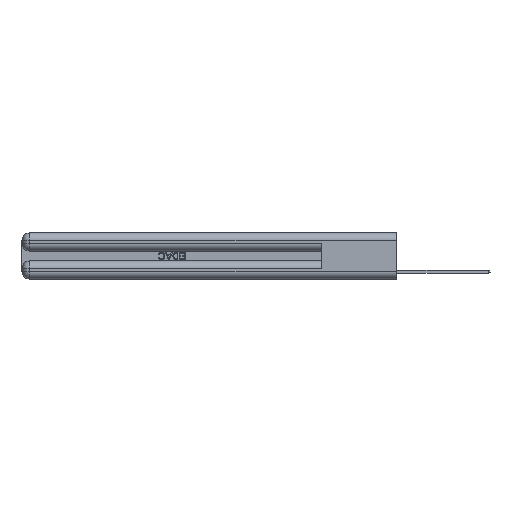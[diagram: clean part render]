
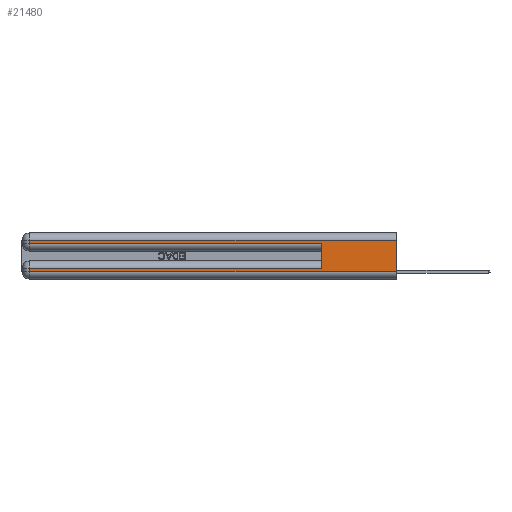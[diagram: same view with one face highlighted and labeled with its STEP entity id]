
A CAD part, left-side view. The second image highlights one B-rep face of the part: STEP entity #21480.
In plain terms, the highlighted planar face has unit normal (-1, 0, 0).
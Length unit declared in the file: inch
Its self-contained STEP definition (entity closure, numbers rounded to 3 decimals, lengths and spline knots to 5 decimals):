
#236 = CARTESIAN_POINT ( 'NONE',  ( 0., 2.94, 0.31 ) ) ;
#272 = EDGE_CURVE ( 'NONE', #16453, #19602, #9130, .T. ) ;
#356 = EDGE_CURVE ( 'NONE', #14904, #26834, #14768, .T. ) ;
#558 = CARTESIAN_POINT ( 'NONE',  ( 0., 0., 0.06 ) ) ;
#974 = VECTOR ( 'NONE', #5524, 39.37008 ) ;
#1012 = LINE ( 'NONE', #23505, #15067 ) ;
#1538 = EDGE_LOOP ( 'NONE', ( #4612, #5909, #6486, #6967, #2007, #4223, #28907, #12622 ) ) ;
#1742 = VECTOR ( 'NONE', #5453, 39.37008 ) ;
#2007 = ORIENTED_EDGE ( 'NONE', *, *, #27892, .F. ) ;
#2695 = VERTEX_POINT ( 'NONE', #4060 ) ;
#4060 = CARTESIAN_POINT ( 'NONE',  ( 0., 0., 0.31 ) ) ;
#4223 = ORIENTED_EDGE ( 'NONE', *, *, #356, .T. ) ;
#4612 = ORIENTED_EDGE ( 'NONE', *, *, #16664, .F. ) ;
#4970 = CARTESIAN_POINT ( 'NONE',  ( 0., 2.94, 0.37 ) ) ;
#5013 = CARTESIAN_POINT ( 'NONE',  ( 0., 0.6, 0.085 ) ) ;
#5196 = EDGE_CURVE ( 'NONE', #2695, #18252, #1012, .T. ) ;
#5453 = DIRECTION ( 'NONE',  ( 0., 0., -1. ) ) ;
#5524 = DIRECTION ( 'NONE',  ( 0., 0., -1. ) ) ;
#5909 = ORIENTED_EDGE ( 'NONE', *, *, #5196, .T. ) ;
#6486 = ORIENTED_EDGE ( 'NONE', *, *, #9444, .T. ) ;
#6498 = LINE ( 'NONE', #16460, #12596 ) ;
#6712 = VERTEX_POINT ( 'NONE', #17236 ) ;
#6967 = ORIENTED_EDGE ( 'NONE', *, *, #272, .T. ) ;
#7532 = CARTESIAN_POINT ( 'NONE',  ( 0., 2.94, 0.37 ) ) ;
#8417 = CARTESIAN_POINT ( 'NONE',  ( 0., 0., 0.37 ) ) ;
#9130 = LINE ( 'NONE', #19065, #28311 ) ;
#9444 = EDGE_CURVE ( 'NONE', #18252, #16453, #19934, .T. ) ;
#9682 = EDGE_CURVE ( 'NONE', #6712, #18373, #23986, .T. ) ;
#10321 = DIRECTION ( 'NONE',  ( 0., 0., -1. ) ) ;
#10399 = DIRECTION ( 'NONE',  ( 0., 0., -1. ) ) ;
#12596 = VECTOR ( 'NONE', #28639, 39.37008 ) ;
#12622 = ORIENTED_EDGE ( 'NONE', *, *, #9682, .T. ) ;
#13651 = LINE ( 'NONE', #8417, #974 ) ;
#14075 = DIRECTION ( 'NONE',  ( 0., -1., 0. ) ) ;
#14768 = LINE ( 'NONE', #22577, #26236 ) ;
#14904 = VERTEX_POINT ( 'NONE', #5013 ) ;
#15067 = VECTOR ( 'NONE', #23666, 39.37008 ) ;
#15297 = PLANE ( 'NONE',  #26217 ) ;
#16453 = VERTEX_POINT ( 'NONE', #26852 ) ;
#16460 = CARTESIAN_POINT ( 'NONE',  ( 0., 0.6, 0.145 ) ) ;
#16664 = EDGE_CURVE ( 'NONE', #2695, #18373, #13651, .T. ) ;
#17236 = CARTESIAN_POINT ( 'NONE',  ( 0., 2.94, 0.06 ) ) ;
#17374 = DIRECTION ( 'NONE',  ( 0., 1., 0. ) ) ;
#18252 = VERTEX_POINT ( 'NONE', #236 ) ;
#18373 = VERTEX_POINT ( 'NONE', #558 ) ;
#18768 = CARTESIAN_POINT ( 'NONE',  ( 0., 0., 0.06 ) ) ;
#19065 = CARTESIAN_POINT ( 'NONE',  ( 0., 0., 0.285 ) ) ;
#19191 = CARTESIAN_POINT ( 'NONE',  ( 0., 2.94, 0.085 ) ) ;
#19602 = VERTEX_POINT ( 'NONE', #20376 ) ;
#19934 = LINE ( 'NONE', #4970, #23677 ) ;
#20376 = CARTESIAN_POINT ( 'NONE',  ( 0., 0.6, 0.285 ) ) ;
#20506 = FACE_OUTER_BOUND ( 'NONE', #1538, .T. ) ;
#20680 = DIRECTION ( 'NONE',  ( 1., 0., 0. ) ) ;
#21480 = ADVANCED_FACE ( 'NONE', ( #20506 ), #15297, .F. ) ;
#22577 = CARTESIAN_POINT ( 'NONE',  ( 0., 0., 0.085 ) ) ;
#23505 = CARTESIAN_POINT ( 'NONE',  ( 0., 0., 0.31 ) ) ;
#23666 = DIRECTION ( 'NONE',  ( 0., 1., 0. ) ) ;
#23677 = VECTOR ( 'NONE', #10321, 39.37008 ) ;
#23986 = LINE ( 'NONE', #18768, #28859 ) ;
#25477 = LINE ( 'NONE', #7532, #1742 ) ;
#26217 = AXIS2_PLACEMENT_3D ( 'NONE', #30427, #20680, #10399 ) ;
#26236 = VECTOR ( 'NONE', #17374, 39.37008 ) ;
#26834 = VERTEX_POINT ( 'NONE', #19191 ) ;
#26852 = CARTESIAN_POINT ( 'NONE',  ( 0., 2.94, 0.285 ) ) ;
#27892 = EDGE_CURVE ( 'NONE', #14904, #19602, #6498, .T. ) ;
#28311 = VECTOR ( 'NONE', #28991, 39.37008 ) ;
#28639 = DIRECTION ( 'NONE',  ( 0., 0., 1. ) ) ;
#28859 = VECTOR ( 'NONE', #14075, 39.37008 ) ;
#28907 = ORIENTED_EDGE ( 'NONE', *, *, #30152, .T. ) ;
#28991 = DIRECTION ( 'NONE',  ( 0., -1., 0. ) ) ;
#30152 = EDGE_CURVE ( 'NONE', #26834, #6712, #25477, .T. ) ;
#30427 = CARTESIAN_POINT ( 'NONE',  ( 0., 0., 0.37 ) ) ;
